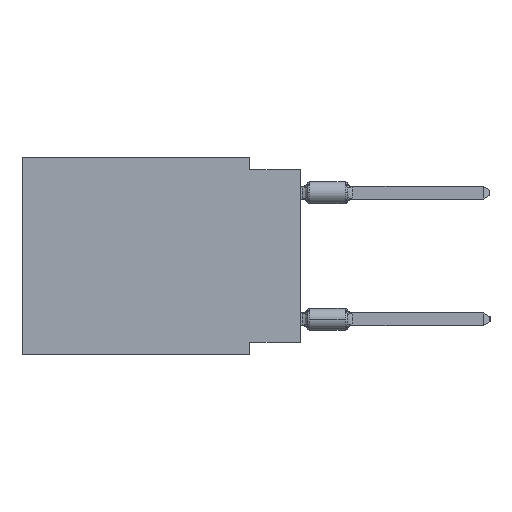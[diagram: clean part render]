
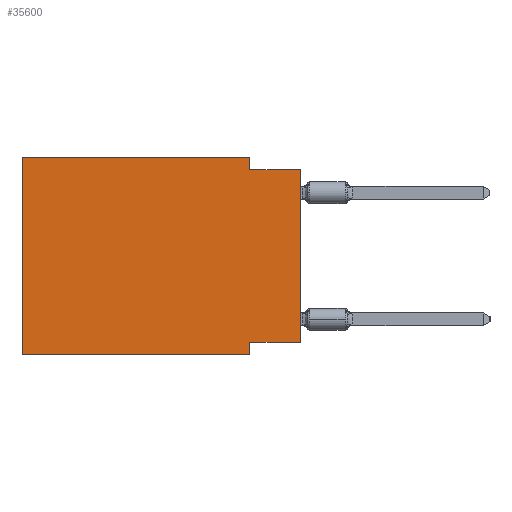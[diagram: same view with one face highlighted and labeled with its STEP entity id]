
A CAD part, left-side view. The second image highlights one B-rep face of the part: STEP entity #35600.
In plain terms, the highlighted planar face has unit normal (-1, 0, 0).
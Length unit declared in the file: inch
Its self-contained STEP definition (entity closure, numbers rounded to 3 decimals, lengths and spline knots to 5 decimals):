
#804 = CARTESIAN_POINT ( 'NONE',  ( 0., 0.55, 0. ) ) ;
#1993 = VERTEX_POINT ( 'NONE', #34829 ) ;
#2205 = CARTESIAN_POINT ( 'NONE',  ( 0., 0.1, -0.365 ) ) ;
#2930 = VECTOR ( 'NONE', #28741, 39.37008 ) ;
#3574 = DIRECTION ( 'NONE',  ( 0., 0., -1. ) ) ;
#4546 = CARTESIAN_POINT ( 'NONE',  ( 0., 0., -0.025 ) ) ;
#4738 = CARTESIAN_POINT ( 'NONE',  ( 0., 0.55, -0.39 ) ) ;
#4926 = DIRECTION ( 'NONE',  ( 0., 0., 1. ) ) ;
#5460 = EDGE_CURVE ( 'NONE', #13670, #26128, #29256, .T. ) ;
#5705 = CARTESIAN_POINT ( 'NONE',  ( 0., 0.55, 0. ) ) ;
#7060 = EDGE_CURVE ( 'NONE', #1993, #12726, #11892, .T. ) ;
#8216 = VERTEX_POINT ( 'NONE', #10713 ) ;
#8830 = ORIENTED_EDGE ( 'NONE', *, *, #18437, .F. ) ;
#9070 = VECTOR ( 'NONE', #3574, 39.37008 ) ;
#9385 = EDGE_CURVE ( 'NONE', #16792, #1993, #27865, .T. ) ;
#9758 = EDGE_CURVE ( 'NONE', #26248, #12726, #30628, .T. ) ;
#10488 = AXIS2_PLACEMENT_3D ( 'NONE', #34555, #31790, #23022 ) ;
#10713 = CARTESIAN_POINT ( 'NONE',  ( 0., 0.55, -0.39 ) ) ;
#11892 = LINE ( 'NONE', #23239, #34200 ) ;
#12195 = CARTESIAN_POINT ( 'NONE',  ( 0., 0.1, 0. ) ) ;
#12291 = CARTESIAN_POINT ( 'NONE',  ( 0., 0.1, -0.39 ) ) ;
#12726 = VERTEX_POINT ( 'NONE', #4546 ) ;
#13670 = VERTEX_POINT ( 'NONE', #2205 ) ;
#14218 = VECTOR ( 'NONE', #4926, 39.37008 ) ;
#14844 = FACE_OUTER_BOUND ( 'NONE', #26174, .T. ) ;
#15237 = CARTESIAN_POINT ( 'NONE',  ( 0., 0.1, -0.39 ) ) ;
#15377 = ORIENTED_EDGE ( 'NONE', *, *, #23733, .T. ) ;
#16792 = VERTEX_POINT ( 'NONE', #12195 ) ;
#16854 = ORIENTED_EDGE ( 'NONE', *, *, #5460, .F. ) ;
#17047 = DIRECTION ( 'NONE',  ( 0., -1., 0. ) ) ;
#17370 = LINE ( 'NONE', #28937, #2930 ) ;
#18437 = EDGE_CURVE ( 'NONE', #8216, #19715, #17370, .T. ) ;
#19278 = CARTESIAN_POINT ( 'NONE',  ( 0., 0., -0.365 ) ) ;
#19715 = VERTEX_POINT ( 'NONE', #804 ) ;
#20791 = LINE ( 'NONE', #5705, #35777 ) ;
#22141 = EDGE_CURVE ( 'NONE', #19715, #16792, #20791, .T. ) ;
#23022 = DIRECTION ( 'NONE',  ( 0., 0., -1. ) ) ;
#23163 = ORIENTED_EDGE ( 'NONE', *, *, #22141, .F. ) ;
#23200 = ORIENTED_EDGE ( 'NONE', *, *, #9385, .F. ) ;
#23239 = CARTESIAN_POINT ( 'NONE',  ( 0., 0., -0.025 ) ) ;
#23733 = EDGE_CURVE ( 'NONE', #8216, #26128, #25020, .T. ) ;
#23807 = DIRECTION ( 'NONE',  ( 0., -1., 0. ) ) ;
#24171 = VECTOR ( 'NONE', #24517, 39.37008 ) ;
#24517 = DIRECTION ( 'NONE',  ( 0., 0., -1. ) ) ;
#24520 = LINE ( 'NONE', #35856, #29398 ) ;
#24888 = CARTESIAN_POINT ( 'NONE',  ( 0., 0.1, 0. ) ) ;
#25020 = LINE ( 'NONE', #4738, #36385 ) ;
#26128 = VERTEX_POINT ( 'NONE', #15237 ) ;
#26174 = EDGE_LOOP ( 'NONE', ( #26246, #29152, #23200, #23163, #8830, #15377, #16854, #34930 ) ) ;
#26246 = ORIENTED_EDGE ( 'NONE', *, *, #9758, .T. ) ;
#26248 = VERTEX_POINT ( 'NONE', #19278 ) ;
#26384 = EDGE_CURVE ( 'NONE', #26248, #13670, #24520, .T. ) ;
#27865 = LINE ( 'NONE', #24888, #24171 ) ;
#28741 = DIRECTION ( 'NONE',  ( 0., 0., 1. ) ) ;
#28937 = CARTESIAN_POINT ( 'NONE',  ( 0., 0.55, 0. ) ) ;
#29152 = ORIENTED_EDGE ( 'NONE', *, *, #7060, .F. ) ;
#29256 = LINE ( 'NONE', #12291, #9070 ) ;
#29398 = VECTOR ( 'NONE', #33080, 39.37008 ) ;
#30444 = CARTESIAN_POINT ( 'NONE',  ( 0., 0., 0. ) ) ;
#30628 = LINE ( 'NONE', #30444, #14218 ) ;
#31790 = DIRECTION ( 'NONE',  ( 1., 0., 0. ) ) ;
#32333 = PLANE ( 'NONE',  #10488 ) ;
#33080 = DIRECTION ( 'NONE',  ( 0., 1., 0. ) ) ;
#34200 = VECTOR ( 'NONE', #23807, 39.37008 ) ;
#34555 = CARTESIAN_POINT ( 'NONE',  ( 0., 0.55, 0. ) ) ;
#34829 = CARTESIAN_POINT ( 'NONE',  ( 0., 0.1, -0.025 ) ) ;
#34930 = ORIENTED_EDGE ( 'NONE', *, *, #26384, .F. ) ;
#35600 = ADVANCED_FACE ( 'NONE', ( #14844 ), #32333, .F. ) ;
#35777 = VECTOR ( 'NONE', #17047, 39.37008 ) ;
#35856 = CARTESIAN_POINT ( 'NONE',  ( 0., 0., -0.365 ) ) ;
#36351 = DIRECTION ( 'NONE',  ( 0., -1., 0. ) ) ;
#36385 = VECTOR ( 'NONE', #36351, 39.37008 ) ;
